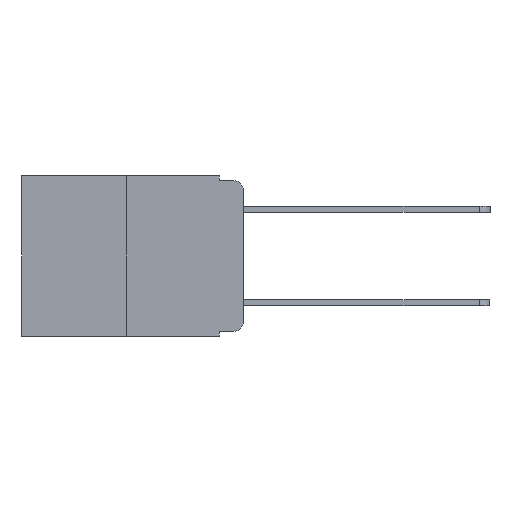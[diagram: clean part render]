
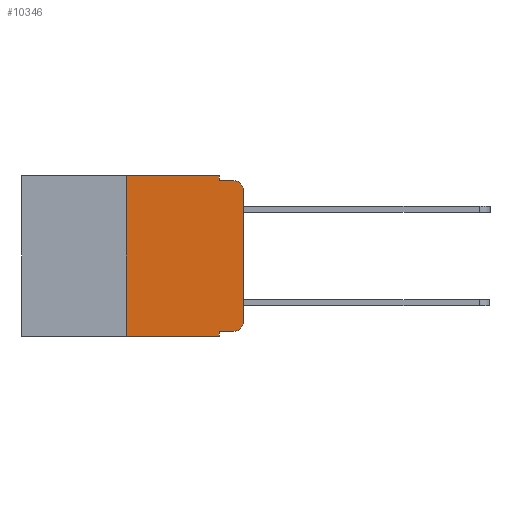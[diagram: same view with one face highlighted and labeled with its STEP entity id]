
A CAD part, left-side view. The second image highlights one B-rep face of the part: STEP entity #10346.
In plain terms, the highlighted planar face has unit normal (-1, 0, 0).
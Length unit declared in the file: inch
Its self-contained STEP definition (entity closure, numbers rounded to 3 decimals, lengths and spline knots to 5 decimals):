
#218 = CARTESIAN_POINT ( 'NONE',  ( 0., 0., -0.313 ) ) ;
#583 = ORIENTED_EDGE ( 'NONE', *, *, #10015, .F. ) ;
#610 = EDGE_CURVE ( 'NONE', #22046, #10748, #21570, .T. ) ;
#754 = VERTEX_POINT ( 'NONE', #22562 ) ;
#934 = ORIENTED_EDGE ( 'NONE', *, *, #3711, .F. ) ;
#1092 = ORIENTED_EDGE ( 'NONE', *, *, #23656, .F. ) ;
#1257 = ORIENTED_EDGE ( 'NONE', *, *, #8124, .T. ) ;
#1294 = ORIENTED_EDGE ( 'NONE', *, *, #610, .T. ) ;
#1297 = EDGE_CURVE ( 'NONE', #14401, #754, #22355, .T. ) ;
#1627 = ORIENTED_EDGE ( 'NONE', *, *, #23766, .F. ) ;
#1816 = ORIENTED_EDGE ( 'NONE', *, *, #22144, .T. ) ;
#2217 = ORIENTED_EDGE ( 'NONE', *, *, #1297, .T. ) ;
#2948 = VECTOR ( 'NONE', #4088, 39.37008 ) ;
#3032 = DIRECTION ( 'NONE',  ( 0., 0., 1. ) ) ;
#3518 = VECTOR ( 'NONE', #5233, 39.37008 ) ;
#3646 = CARTESIAN_POINT ( 'NONE',  ( 0., 0.051, 0. ) ) ;
#3711 = EDGE_CURVE ( 'NONE', #15089, #16690, #6022, .T. ) ;
#3716 = DIRECTION ( 'NONE',  ( -1., 0., 0. ) ) ;
#3940 = ORIENTED_EDGE ( 'NONE', *, *, #21399, .F. ) ;
#4065 = CARTESIAN_POINT ( 'NONE',  ( 0., 0.051, 0. ) ) ;
#4088 = DIRECTION ( 'NONE',  ( 0., -1., 0. ) ) ;
#4209 = LINE ( 'NONE', #4065, #13524 ) ;
#5054 = VECTOR ( 'NONE', #11897, 39.37008 ) ;
#5233 = DIRECTION ( 'NONE',  ( 0., -1., 0. ) ) ;
#5855 = ORIENTED_EDGE ( 'NONE', *, *, #14279, .T. ) ;
#6022 = LINE ( 'NONE', #3646, #15828 ) ;
#6347 = DIRECTION ( 'NONE',  ( -1., 0., 0. ) ) ;
#6467 = FACE_OUTER_BOUND ( 'NONE', #6837, .T. ) ;
#6567 = VERTEX_POINT ( 'NONE', #21362 ) ;
#6837 = EDGE_LOOP ( 'NONE', ( #1294, #1816, #583, #934, #1092, #1627, #2217, #3940, #5855, #1257 ) ) ;
#7050 = VECTOR ( 'NONE', #3032, 39.37008 ) ;
#7088 = CARTESIAN_POINT ( 'NONE',  ( 0., 0.25, 0. ) ) ;
#7855 = CARTESIAN_POINT ( 'NONE',  ( 0., 0.051, -0.01 ) ) ;
#8095 = CARTESIAN_POINT ( 'NONE',  ( 0., 0., 0. ) ) ;
#8100 = DIRECTION ( 'NONE',  ( 1., 0., 0. ) ) ;
#8124 = EDGE_CURVE ( 'NONE', #18243, #22046, #9240, .T. ) ;
#8564 = LINE ( 'NONE', #21600, #3518 ) ;
#8604 = LINE ( 'NONE', #17026, #2948 ) ;
#9240 = CIRCLE ( 'NONE', #14633, 0.02 ) ;
#10010 = LINE ( 'NONE', #22683, #5054 ) ;
#10015 = EDGE_CURVE ( 'NONE', #16690, #6567, #8564, .T. ) ;
#10304 = CIRCLE ( 'NONE', #17219, 0.02 ) ;
#10346 = ADVANCED_FACE ( 'NONE', ( #6467 ), #15394, .F. ) ;
#10748 = VERTEX_POINT ( 'NONE', #16661 ) ;
#11897 = DIRECTION ( 'NONE',  ( 0., 0., 1. ) ) ;
#12555 = AXIS2_PLACEMENT_3D ( 'NONE', #19045, #8100, #20805 ) ;
#12807 = VECTOR ( 'NONE', #13409, 39.37008 ) ;
#13302 = CARTESIAN_POINT ( 'NONE',  ( 0., 0.473, -0.343 ) ) ;
#13388 = CARTESIAN_POINT ( 'NONE',  ( 0., 0.051, -0.333 ) ) ;
#13409 = DIRECTION ( 'NONE',  ( 0., -1., 0. ) ) ;
#13524 = VECTOR ( 'NONE', #15175, 39.37008 ) ;
#14279 = EDGE_CURVE ( 'NONE', #16653, #18243, #17131, .T. ) ;
#14401 = VERTEX_POINT ( 'NONE', #15595 ) ;
#14633 = AXIS2_PLACEMENT_3D ( 'NONE', #14858, #3716, #16693 ) ;
#14858 = CARTESIAN_POINT ( 'NONE',  ( 0., 0.02, -0.313 ) ) ;
#15089 = VERTEX_POINT ( 'NONE', #18225 ) ;
#15175 = DIRECTION ( 'NONE',  ( 0., 0., -1. ) ) ;
#15205 = DIRECTION ( 'NONE',  ( 0., -1., 0. ) ) ;
#15394 = PLANE ( 'NONE',  #12555 ) ;
#15595 = CARTESIAN_POINT ( 'NONE',  ( 0., 0.25, -0.343 ) ) ;
#15828 = VECTOR ( 'NONE', #16625, 39.37008 ) ;
#16625 = DIRECTION ( 'NONE',  ( 0., 0., -1. ) ) ;
#16653 = VERTEX_POINT ( 'NONE', #22342 ) ;
#16661 = CARTESIAN_POINT ( 'NONE',  ( 0., 0., -0.03 ) ) ;
#16690 = VERTEX_POINT ( 'NONE', #7855 ) ;
#16693 = DIRECTION ( 'NONE',  ( 0., 0., -1. ) ) ;
#17026 = CARTESIAN_POINT ( 'NONE',  ( 0., 0.473, 0. ) ) ;
#17131 = LINE ( 'NONE', #13388, #21320 ) ;
#17219 = AXIS2_PLACEMENT_3D ( 'NONE', #17345, #6347, #19182 ) ;
#17345 = CARTESIAN_POINT ( 'NONE',  ( 0., 0.02, -0.03 ) ) ;
#17737 = CARTESIAN_POINT ( 'NONE',  ( 0., 0.02, -0.333 ) ) ;
#18225 = CARTESIAN_POINT ( 'NONE',  ( 0., 0.051, 0. ) ) ;
#18243 = VERTEX_POINT ( 'NONE', #17737 ) ;
#19045 = CARTESIAN_POINT ( 'NONE',  ( 0., 0.473, 0. ) ) ;
#19182 = DIRECTION ( 'NONE',  ( 0., 0., -1. ) ) ;
#20805 = DIRECTION ( 'NONE',  ( 0., 0., -1. ) ) ;
#21320 = VECTOR ( 'NONE', #15205, 39.37008 ) ;
#21362 = CARTESIAN_POINT ( 'NONE',  ( 0., 0.02, -0.01 ) ) ;
#21399 = EDGE_CURVE ( 'NONE', #16653, #754, #4209, .T. ) ;
#21570 = LINE ( 'NONE', #8095, #7050 ) ;
#21600 = CARTESIAN_POINT ( 'NONE',  ( 0., 0.051, -0.01 ) ) ;
#22046 = VERTEX_POINT ( 'NONE', #218 ) ;
#22144 = EDGE_CURVE ( 'NONE', #10748, #6567, #10304, .T. ) ;
#22342 = CARTESIAN_POINT ( 'NONE',  ( 0., 0.051, -0.333 ) ) ;
#22355 = LINE ( 'NONE', #13302, #12807 ) ;
#22387 = VERTEX_POINT ( 'NONE', #7088 ) ;
#22562 = CARTESIAN_POINT ( 'NONE',  ( 0., 0.051, -0.343 ) ) ;
#22683 = CARTESIAN_POINT ( 'NONE',  ( 0., 0.25, 0. ) ) ;
#23656 = EDGE_CURVE ( 'NONE', #22387, #15089, #8604, .T. ) ;
#23766 = EDGE_CURVE ( 'NONE', #14401, #22387, #10010, .T. ) ;
